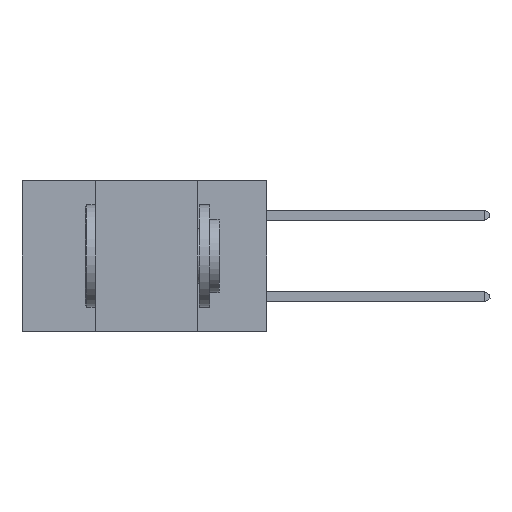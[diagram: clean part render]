
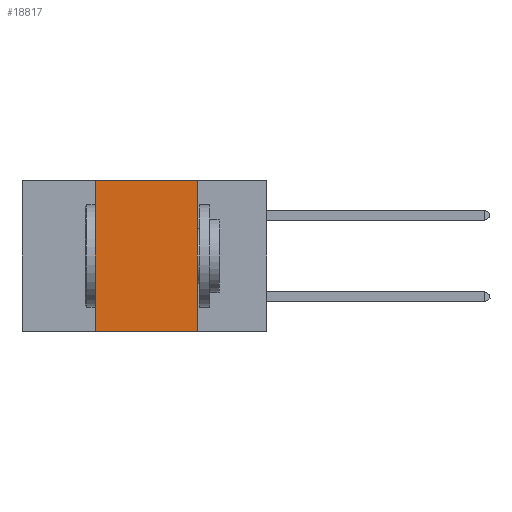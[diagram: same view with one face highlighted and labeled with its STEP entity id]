
A CAD part, left-side view. The second image highlights one B-rep face of the part: STEP entity #18817.
In plain terms, the highlighted planar face has unit normal (-1, 0, 0).
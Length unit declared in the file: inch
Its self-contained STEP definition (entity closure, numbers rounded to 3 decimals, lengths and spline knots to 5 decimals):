
#548 = VECTOR ( 'NONE', #21975, 39.37008 ) ;
#789 = VECTOR ( 'NONE', #6490, 39.37008 ) ;
#865 = CARTESIAN_POINT ( 'NONE',  ( 0., 0.42, -0.37 ) ) ;
#2463 = EDGE_LOOP ( 'NONE', ( #8545, #10877, #12265, #4442 ) ) ;
#3489 = EDGE_CURVE ( 'NONE', #22808, #9484, #6180, .T. ) ;
#4442 = ORIENTED_EDGE ( 'NONE', *, *, #11041, .T. ) ;
#5950 = VECTOR ( 'NONE', #14048, 39.37008 ) ;
#6180 = LINE ( 'NONE', #10620, #789 ) ;
#6299 = PLANE ( 'NONE',  #14812 ) ;
#6466 = CARTESIAN_POINT ( 'NONE',  ( 0., 0.17, 0. ) ) ;
#6490 = DIRECTION ( 'NONE',  ( 0., 0., 1. ) ) ;
#7479 = CARTESIAN_POINT ( 'NONE',  ( 0., 0.6, -0.37 ) ) ;
#7727 = FACE_OUTER_BOUND ( 'NONE', #2463, .T. ) ;
#8545 = ORIENTED_EDGE ( 'NONE', *, *, #9707, .F. ) ;
#9484 = VERTEX_POINT ( 'NONE', #12479 ) ;
#9707 = EDGE_CURVE ( 'NONE', #18912, #22396, #12500, .T. ) ;
#10261 = CARTESIAN_POINT ( 'NONE',  ( 0., 0.6, 0. ) ) ;
#10620 = CARTESIAN_POINT ( 'NONE',  ( 0., 0.42, 0. ) ) ;
#10877 = ORIENTED_EDGE ( 'NONE', *, *, #18609, .F. ) ;
#10907 = CARTESIAN_POINT ( 'NONE',  ( 0., 0.17, -0.37 ) ) ;
#10997 = LINE ( 'NONE', #15879, #5950 ) ;
#11041 = EDGE_CURVE ( 'NONE', #22808, #22396, #14300, .T. ) ;
#11255 = DIRECTION ( 'NONE',  ( 0., -1., 0. ) ) ;
#12265 = ORIENTED_EDGE ( 'NONE', *, *, #3489, .F. ) ;
#12479 = CARTESIAN_POINT ( 'NONE',  ( 0., 0.42, 0. ) ) ;
#12500 = LINE ( 'NONE', #21801, #548 ) ;
#14048 = DIRECTION ( 'NONE',  ( 0., -1., 0. ) ) ;
#14300 = LINE ( 'NONE', #7479, #15506 ) ;
#14812 = AXIS2_PLACEMENT_3D ( 'NONE', #10261, #15778, #19737 ) ;
#15506 = VECTOR ( 'NONE', #11255, 39.37008 ) ;
#15778 = DIRECTION ( 'NONE',  ( 1., 0., 0. ) ) ;
#15879 = CARTESIAN_POINT ( 'NONE',  ( 0., 0.6, 0. ) ) ;
#18609 = EDGE_CURVE ( 'NONE', #9484, #18912, #10997, .T. ) ;
#18817 = ADVANCED_FACE ( 'NONE', ( #7727 ), #6299, .F. ) ;
#18912 = VERTEX_POINT ( 'NONE', #6466 ) ;
#19737 = DIRECTION ( 'NONE',  ( 0., 0., -1. ) ) ;
#21801 = CARTESIAN_POINT ( 'NONE',  ( 0., 0.17, 0. ) ) ;
#21975 = DIRECTION ( 'NONE',  ( 0., 0., -1. ) ) ;
#22396 = VERTEX_POINT ( 'NONE', #10907 ) ;
#22808 = VERTEX_POINT ( 'NONE', #865 ) ;
